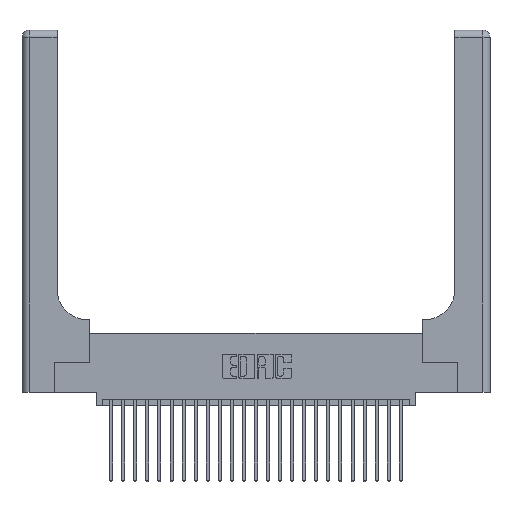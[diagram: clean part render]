
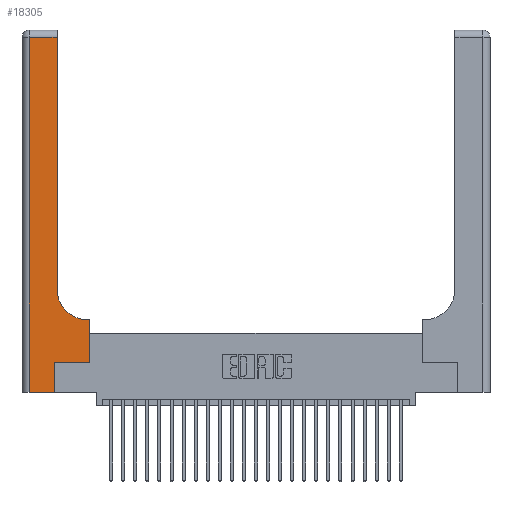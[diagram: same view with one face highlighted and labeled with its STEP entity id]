
A CAD part, top view. The second image highlights one B-rep face of the part: STEP entity #18305.
In plain terms, the highlighted planar face has unit normal (0, 0, 1).
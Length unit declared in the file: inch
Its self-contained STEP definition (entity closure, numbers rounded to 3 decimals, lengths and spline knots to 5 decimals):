
#94 = CARTESIAN_POINT ( 'NONE',  ( 0.269, 0., 0.37 ) ) ;
#305 = CARTESIAN_POINT ( 'NONE',  ( 0.269, 0.25, 0.37 ) ) ;
#715 = VECTOR ( 'NONE', #21260, 39.37008 ) ;
#728 = CARTESIAN_POINT ( 'NONE',  ( 0., 2.94, 0.37 ) ) ;
#1104 = FACE_OUTER_BOUND ( 'NONE', #25993, .T. ) ;
#1332 = CARTESIAN_POINT ( 'NONE',  ( 0.2915, 0.85, 0.37 ) ) ;
#1479 = EDGE_CURVE ( 'NONE', #10934, #19488, #9637, .T. ) ;
#1960 = LINE ( 'NONE', #19017, #23642 ) ;
#2152 = VERTEX_POINT ( 'NONE', #26277 ) ;
#2264 = VERTEX_POINT ( 'NONE', #20474 ) ;
#2606 = ORIENTED_EDGE ( 'NONE', *, *, #19969, .T. ) ;
#2940 = CARTESIAN_POINT ( 'NONE',  ( 0.2915, 0.6, 0.37 ) ) ;
#3332 = LINE ( 'NONE', #8102, #15125 ) ;
#3482 = CARTESIAN_POINT ( 'NONE',  ( 0.5415, 0.85, 0.37 ) ) ;
#4145 = ORIENTED_EDGE ( 'NONE', *, *, #26624, .T. ) ;
#4190 = DIRECTION ( 'NONE',  ( 0., 1., 0. ) ) ;
#4527 = EDGE_CURVE ( 'NONE', #15363, #12683, #18013, .T. ) ;
#4870 = DIRECTION ( 'NONE',  ( 0., 0., -1. ) ) ;
#5210 = AXIS2_PLACEMENT_3D ( 'NONE', #3482, #26600, #22379 ) ;
#5300 = EDGE_CURVE ( 'NONE', #12012, #15363, #8444, .T. ) ;
#5487 = ORIENTED_EDGE ( 'NONE', *, *, #20708, .T. ) ;
#5629 = ORIENTED_EDGE ( 'NONE', *, *, #8536, .T. ) ;
#7163 = ORIENTED_EDGE ( 'NONE', *, *, #1479, .T. ) ;
#7249 = ORIENTED_EDGE ( 'NONE', *, *, #11881, .T. ) ;
#7325 = AXIS2_PLACEMENT_3D ( 'NONE', #23497, #4870, #11188 ) ;
#7769 = VECTOR ( 'NONE', #13417, 39.37008 ) ;
#8102 = CARTESIAN_POINT ( 'NONE',  ( 0., 0., 0.37 ) ) ;
#8444 = LINE ( 'NONE', #2940, #16954 ) ;
#8536 = EDGE_CURVE ( 'NONE', #2264, #19799, #19711, .T. ) ;
#9259 = VERTEX_POINT ( 'NONE', #16393 ) ;
#9637 = LINE ( 'NONE', #12805, #715 ) ;
#9901 = LINE ( 'NONE', #25991, #10544 ) ;
#9947 = CARTESIAN_POINT ( 'NONE',  ( 0.5585, 0.6, 0.37 ) ) ;
#10544 = VECTOR ( 'NONE', #17721, 39.37008 ) ;
#10934 = VERTEX_POINT ( 'NONE', #24623 ) ;
#10995 = CARTESIAN_POINT ( 'NONE',  ( 0.5415, 0.6, 0.37 ) ) ;
#11188 = DIRECTION ( 'NONE',  ( -1., 0., 0. ) ) ;
#11881 = EDGE_CURVE ( 'NONE', #2152, #10934, #12360, .T. ) ;
#12012 = VERTEX_POINT ( 'NONE', #9947 ) ;
#12360 = LINE ( 'NONE', #728, #7769 ) ;
#12683 = VERTEX_POINT ( 'NONE', #1332 ) ;
#12805 = CARTESIAN_POINT ( 'NONE',  ( 0.06, 3., 0.37 ) ) ;
#12946 = DIRECTION ( 'NONE',  ( 0., 1., 0. ) ) ;
#13105 = PLANE ( 'NONE',  #7325 ) ;
#13417 = DIRECTION ( 'NONE',  ( -1., 0., 0. ) ) ;
#14173 = ORIENTED_EDGE ( 'NONE', *, *, #4527, .T. ) ;
#14546 = CARTESIAN_POINT ( 'NONE',  ( 0.06, 0., 0.37 ) ) ;
#14936 = DIRECTION ( 'NONE',  ( 1., 0., 0. ) ) ;
#15125 = VECTOR ( 'NONE', #16365, 39.37008 ) ;
#15363 = VERTEX_POINT ( 'NONE', #10995 ) ;
#15699 = VECTOR ( 'NONE', #4190, 39.37008 ) ;
#16238 = EDGE_CURVE ( 'NONE', #9259, #2264, #21278, .T. ) ;
#16365 = DIRECTION ( 'NONE',  ( 1., 0., 0. ) ) ;
#16393 = CARTESIAN_POINT ( 'NONE',  ( 0.269, 0., 0.37 ) ) ;
#16954 = VECTOR ( 'NONE', #24328, 39.37008 ) ;
#17721 = DIRECTION ( 'NONE',  ( 0., 1., 0. ) ) ;
#18013 = CIRCLE ( 'NONE', #5210, 0.25 ) ;
#18305 = ADVANCED_FACE ( 'NONE', ( #1104 ), #13105, .F. ) ;
#18747 = VECTOR ( 'NONE', #14936, 39.37008 ) ;
#19017 = CARTESIAN_POINT ( 'NONE',  ( 0.2915, 3., 0.37 ) ) ;
#19488 = VERTEX_POINT ( 'NONE', #14546 ) ;
#19711 = LINE ( 'NONE', #305, #18747 ) ;
#19799 = VERTEX_POINT ( 'NONE', #19907 ) ;
#19907 = CARTESIAN_POINT ( 'NONE',  ( 0.5585, 0.25, 0.37 ) ) ;
#19969 = EDGE_CURVE ( 'NONE', #19488, #9259, #3332, .T. ) ;
#20065 = ORIENTED_EDGE ( 'NONE', *, *, #16238, .T. ) ;
#20466 = ORIENTED_EDGE ( 'NONE', *, *, #5300, .T. ) ;
#20474 = CARTESIAN_POINT ( 'NONE',  ( 0.269, 0.25, 0.37 ) ) ;
#20708 = EDGE_CURVE ( 'NONE', #12683, #2152, #1960, .T. ) ;
#21260 = DIRECTION ( 'NONE',  ( 0., -1., 0. ) ) ;
#21278 = LINE ( 'NONE', #94, #15699 ) ;
#22379 = DIRECTION ( 'NONE',  ( 1., 0., 0. ) ) ;
#23497 = CARTESIAN_POINT ( 'NONE',  ( 0., 3., 0.37 ) ) ;
#23642 = VECTOR ( 'NONE', #12946, 39.37008 ) ;
#24328 = DIRECTION ( 'NONE',  ( -1., 0., 0. ) ) ;
#24623 = CARTESIAN_POINT ( 'NONE',  ( 0.06, 2.94, 0.37 ) ) ;
#25991 = CARTESIAN_POINT ( 'NONE',  ( 0.5585, 0.25, 0.37 ) ) ;
#25993 = EDGE_LOOP ( 'NONE', ( #5487, #7249, #7163, #2606, #20065, #5629, #4145, #20466, #14173 ) ) ;
#26277 = CARTESIAN_POINT ( 'NONE',  ( 0.2915, 2.94, 0.37 ) ) ;
#26600 = DIRECTION ( 'NONE',  ( 0., 0., -1. ) ) ;
#26624 = EDGE_CURVE ( 'NONE', #19799, #12012, #9901, .T. ) ;
